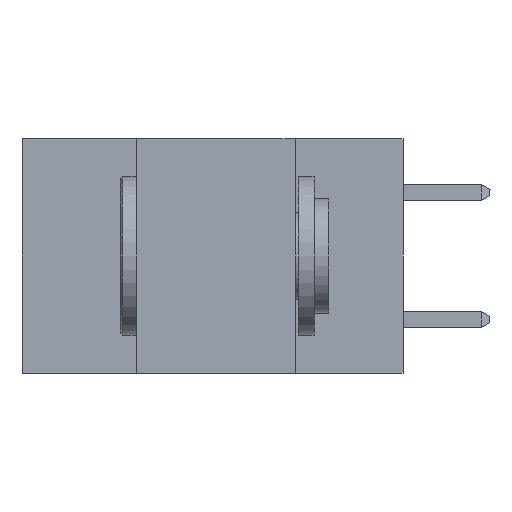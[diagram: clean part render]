
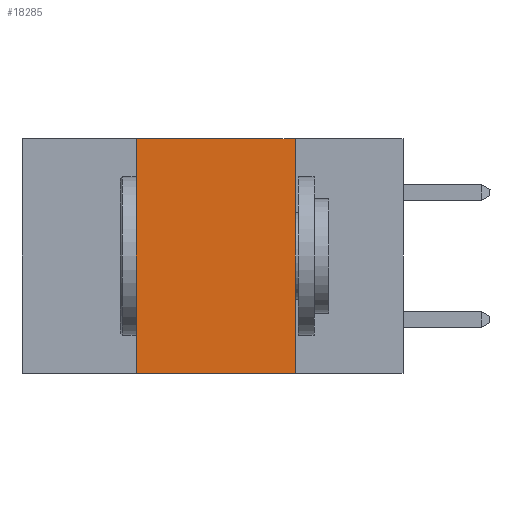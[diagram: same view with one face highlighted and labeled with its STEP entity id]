
A CAD part, left-side view. The second image highlights one B-rep face of the part: STEP entity #18285.
In plain terms, the highlighted planar face has unit normal (-1, 0, 0).
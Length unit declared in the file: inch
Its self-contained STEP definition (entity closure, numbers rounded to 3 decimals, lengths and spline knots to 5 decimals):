
#641 = CARTESIAN_POINT ( 'NONE',  ( 0., 0.42, 0. ) ) ;
#871 = FACE_OUTER_BOUND ( 'NONE', #5295, .T. ) ;
#959 = DIRECTION ( 'NONE',  ( 0., 0., -1. ) ) ;
#1378 = VECTOR ( 'NONE', #6885, 39.37008 ) ;
#1624 = CARTESIAN_POINT ( 'NONE',  ( 0., 0.42, -0.37 ) ) ;
#2454 = CARTESIAN_POINT ( 'NONE',  ( 0., 0.17, 0. ) ) ;
#4707 = CARTESIAN_POINT ( 'NONE',  ( 0., 0.6, 0. ) ) ;
#5243 = LINE ( 'NONE', #20118, #1378 ) ;
#5295 = EDGE_LOOP ( 'NONE', ( #18676, #24641, #7087, #12716 ) ) ;
#5388 = LINE ( 'NONE', #15050, #14601 ) ;
#5509 = DIRECTION ( 'NONE',  ( 0., -1., 0. ) ) ;
#5544 = DIRECTION ( 'NONE',  ( 0., 0., -1. ) ) ;
#6885 = DIRECTION ( 'NONE',  ( 0., 0., 1. ) ) ;
#7087 = ORIENTED_EDGE ( 'NONE', *, *, #20413, .F. ) ;
#7444 = VERTEX_POINT ( 'NONE', #2454 ) ;
#9473 = VERTEX_POINT ( 'NONE', #641 ) ;
#11498 = VERTEX_POINT ( 'NONE', #1624 ) ;
#11550 = EDGE_CURVE ( 'NONE', #9473, #7444, #21443, .T. ) ;
#12716 = ORIENTED_EDGE ( 'NONE', *, *, #15975, .T. ) ;
#13122 = CARTESIAN_POINT ( 'NONE',  ( 0., 0.6, 0. ) ) ;
#14067 = VERTEX_POINT ( 'NONE', #24402 ) ;
#14601 = VECTOR ( 'NONE', #5544, 39.37008 ) ;
#15050 = CARTESIAN_POINT ( 'NONE',  ( 0., 0.17, 0. ) ) ;
#15975 = EDGE_CURVE ( 'NONE', #11498, #14067, #16440, .T. ) ;
#16171 = PLANE ( 'NONE',  #21674 ) ;
#16440 = LINE ( 'NONE', #24109, #19461 ) ;
#18196 = VECTOR ( 'NONE', #5509, 39.37008 ) ;
#18285 = ADVANCED_FACE ( 'NONE', ( #871 ), #16171, .F. ) ;
#18676 = ORIENTED_EDGE ( 'NONE', *, *, #22627, .F. ) ;
#19461 = VECTOR ( 'NONE', #20447, 39.37008 ) ;
#20118 = CARTESIAN_POINT ( 'NONE',  ( 0., 0.42, 0. ) ) ;
#20413 = EDGE_CURVE ( 'NONE', #11498, #9473, #5243, .T. ) ;
#20447 = DIRECTION ( 'NONE',  ( 0., -1., 0. ) ) ;
#21443 = LINE ( 'NONE', #13122, #18196 ) ;
#21674 = AXIS2_PLACEMENT_3D ( 'NONE', #4707, #21854, #959 ) ;
#21854 = DIRECTION ( 'NONE',  ( 1., 0., 0. ) ) ;
#22627 = EDGE_CURVE ( 'NONE', #7444, #14067, #5388, .T. ) ;
#24109 = CARTESIAN_POINT ( 'NONE',  ( 0., 0.6, -0.37 ) ) ;
#24402 = CARTESIAN_POINT ( 'NONE',  ( 0., 0.17, -0.37 ) ) ;
#24641 = ORIENTED_EDGE ( 'NONE', *, *, #11550, .F. ) ;
